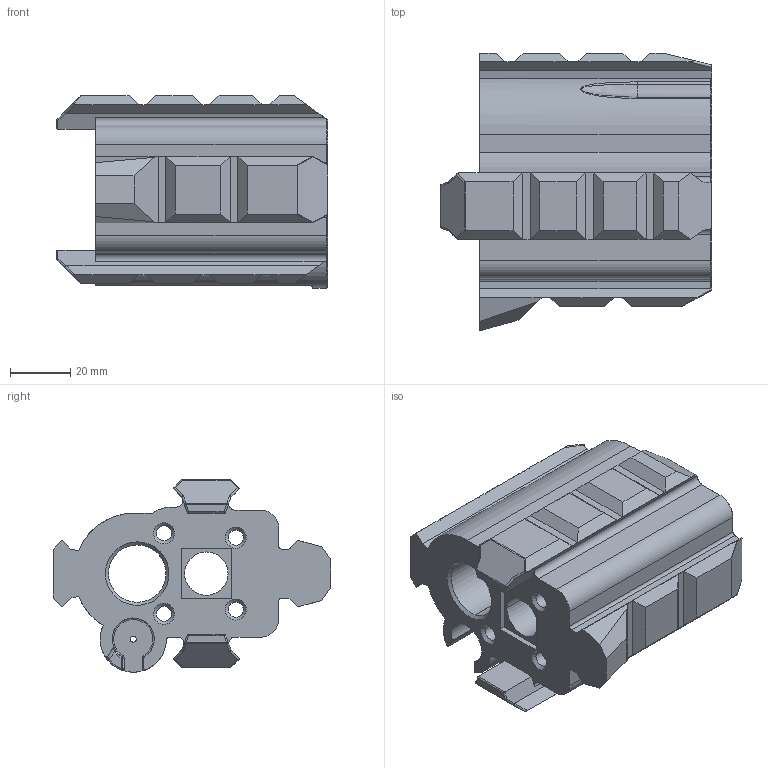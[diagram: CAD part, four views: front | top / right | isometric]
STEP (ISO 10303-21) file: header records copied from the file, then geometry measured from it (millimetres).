
FILE_DESCRIPTION (( 'STEP AP203' ), '1' );
FILE_NAME ('MOD9_barrel_retainer.STEP', '2020-06-10T04:55:25', ( '' ), ( '' ), 'SwSTEP 2.0', 'SolidWorks 2016', '' );
FILE_SCHEMA (( 'CONFIG_CONTROL_DESIGN' ));
Length unit declared in the file: millimetre
Products named in the file (1): MOD9_barrel_retainer
Bounding box: 90.02 x 92.13 x 63.85 mm (x, y, z)
Volume: 158242.5 mm3; surface area: 45990.6 mm2
Topology: 1 solids, 1 shells, 294 faces, 747 edges, 454 vertices
Faces by surface type: plane 147, cylinder 85, cone 43, bspline 8, sphere 6, torus 5
Full cylindrical faces by diameter (mm): 2 x1, 5 x4
Entity records: 9138 total; most frequent: CARTESIAN_POINT 2190, ORIENTED_EDGE 1462, DIRECTION 1387, EDGE_CURVE 731, VECTOR 477, LINE 477, AXIS2_PLACEMENT_3D 455, VERTEX_POINT 452
